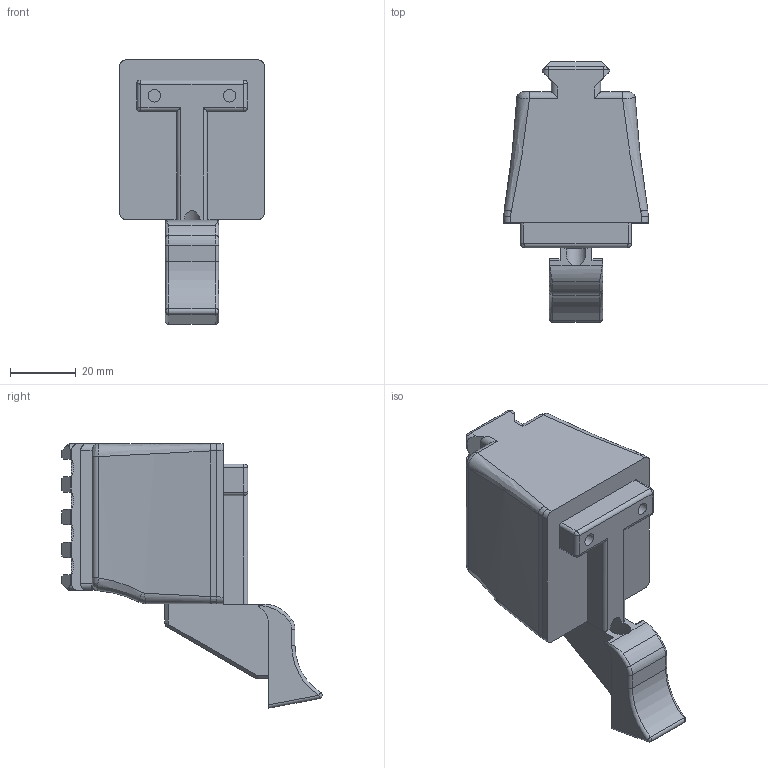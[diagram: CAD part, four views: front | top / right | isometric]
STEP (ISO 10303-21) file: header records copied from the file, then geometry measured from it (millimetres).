
FILE_DESCRIPTION(/* description */ (''),/* implementation_level */ '2;1');
FILE_NAME(/* name */ 'Rear Chassis, Picatinny.step',/* time_stamp */ '2021-08-06T21:53:09-04:00',/* author */ (''),/* organization */ (''),/* preprocessor_version */ 'ST-DEVELOPER v18.1',/* originating_system */ 'Autodesk Translation Framework v10.9.0.1377',/* authorisation */ '');
FILE_SCHEMA (('AUTOMOTIVE_DESIGN { 1 0 10303 214 3 1 1 }'));
Length unit declared in the file: millimetre
Products named in the file (1): Rear Chassis, Picatinny
Bounding box: 44.15 x 79.45 x 80.7 mm (x, y, z)
Volume: 66218.6 mm3; surface area: 21915.6 mm2
Topology: 1 solids, 2 shells, 254 faces, 628 edges, 379 vertices
Faces by surface type: plane 98, cylinder 84, bspline 36, torus 24, sphere 8, cone 4
Full cylindrical faces by diameter (mm): 3.8 x2, 6.097 x1, 20.317 x1, 23.683 x1
Entity records: 8916 total; most frequent: CARTESIAN_POINT 3007, ORIENTED_EDGE 1248, DIRECTION 1205, EDGE_CURVE 624, AXIS2_PLACEMENT_3D 447, VERTEX_POINT 379, LINE 311, VECTOR 311
